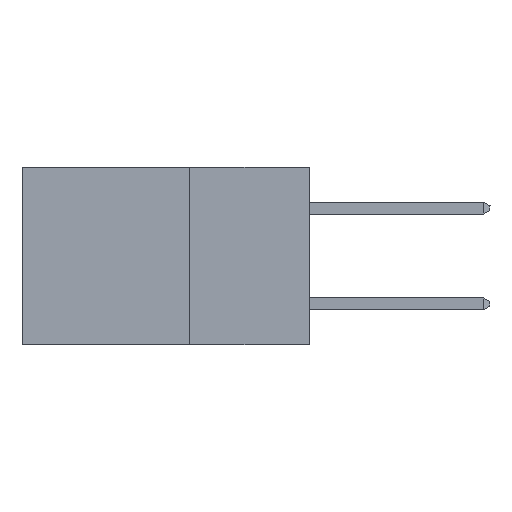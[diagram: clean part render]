
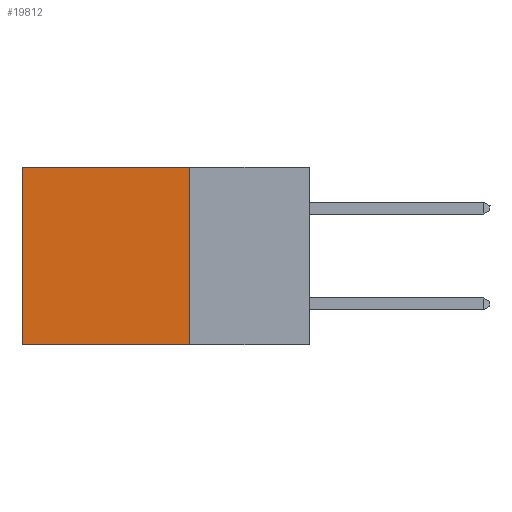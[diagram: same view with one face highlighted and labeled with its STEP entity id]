
A CAD part, left-side view. The second image highlights one B-rep face of the part: STEP entity #19812.
In plain terms, the highlighted planar face has unit normal (-1, 0, 0).
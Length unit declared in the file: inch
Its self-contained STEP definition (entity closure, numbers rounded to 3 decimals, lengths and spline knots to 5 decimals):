
#746 = CARTESIAN_POINT ( 'NONE',  ( 0.2875, 0.25, -0.37 ) ) ;
#3291 = CARTESIAN_POINT ( 'NONE',  ( 0.2875, 0.25, 0. ) ) ;
#3292 = VERTEX_POINT ( 'NONE', #8513 ) ;
#4353 = PLANE ( 'NONE',  #14345 ) ;
#4936 = CARTESIAN_POINT ( 'NONE',  ( 0.2875, 0.25, 0. ) ) ;
#5348 = CARTESIAN_POINT ( 'NONE',  ( 0.2875, 0.25, -0.37 ) ) ;
#8513 = CARTESIAN_POINT ( 'NONE',  ( 0.2875, 0.25, 0. ) ) ;
#9033 = FACE_OUTER_BOUND ( 'NONE', #14852, .T. ) ;
#9590 = VECTOR ( 'NONE', #13685, 39.37008 ) ;
#10021 = VECTOR ( 'NONE', #21492, 39.37008 ) ;
#10275 = EDGE_CURVE ( 'NONE', #3292, #10921, #23003, .T. ) ;
#10921 = VERTEX_POINT ( 'NONE', #746 ) ;
#11251 = VECTOR ( 'NONE', #20808, 39.37008 ) ;
#13685 = DIRECTION ( 'NONE',  ( 0., 1., 0. ) ) ;
#14093 = DIRECTION ( 'NONE',  ( 0., 1., 0. ) ) ;
#14344 = VECTOR ( 'NONE', #14093, 39.37008 ) ;
#14345 = AXIS2_PLACEMENT_3D ( 'NONE', #17912, #22165, #15142 ) ;
#14852 = EDGE_LOOP ( 'NONE', ( #22154, #17820, #21706, #25850 ) ) ;
#14960 = CARTESIAN_POINT ( 'NONE',  ( 0.2875, 0.6, -0.37 ) ) ;
#15142 = DIRECTION ( 'NONE',  ( 0., 0., -1. ) ) ;
#15762 = EDGE_CURVE ( 'NONE', #19916, #27655, #23533, .T. ) ;
#16475 = EDGE_CURVE ( 'NONE', #3292, #19916, #27688, .T. ) ;
#16572 = LINE ( 'NONE', #5348, #14344 ) ;
#17820 = ORIENTED_EDGE ( 'NONE', *, *, #28857, .F. ) ;
#17912 = CARTESIAN_POINT ( 'NONE',  ( 0.2875, 0.25, 0. ) ) ;
#19812 = ADVANCED_FACE ( 'NONE', ( #9033 ), #4353, .F. ) ;
#19916 = VERTEX_POINT ( 'NONE', #20404 ) ;
#20404 = CARTESIAN_POINT ( 'NONE',  ( 0.2875, 0.6, 0. ) ) ;
#20808 = DIRECTION ( 'NONE',  ( 0., 0., -1. ) ) ;
#21492 = DIRECTION ( 'NONE',  ( 0., 0., -1. ) ) ;
#21706 = ORIENTED_EDGE ( 'NONE', *, *, #10275, .F. ) ;
#22154 = ORIENTED_EDGE ( 'NONE', *, *, #15762, .T. ) ;
#22165 = DIRECTION ( 'NONE',  ( 1., 0., 0. ) ) ;
#23003 = LINE ( 'NONE', #3291, #11251 ) ;
#23533 = LINE ( 'NONE', #28086, #10021 ) ;
#25850 = ORIENTED_EDGE ( 'NONE', *, *, #16475, .T. ) ;
#27655 = VERTEX_POINT ( 'NONE', #14960 ) ;
#27688 = LINE ( 'NONE', #4936, #9590 ) ;
#28086 = CARTESIAN_POINT ( 'NONE',  ( 0.2875, 0.6, 0. ) ) ;
#28857 = EDGE_CURVE ( 'NONE', #10921, #27655, #16572, .T. ) ;
